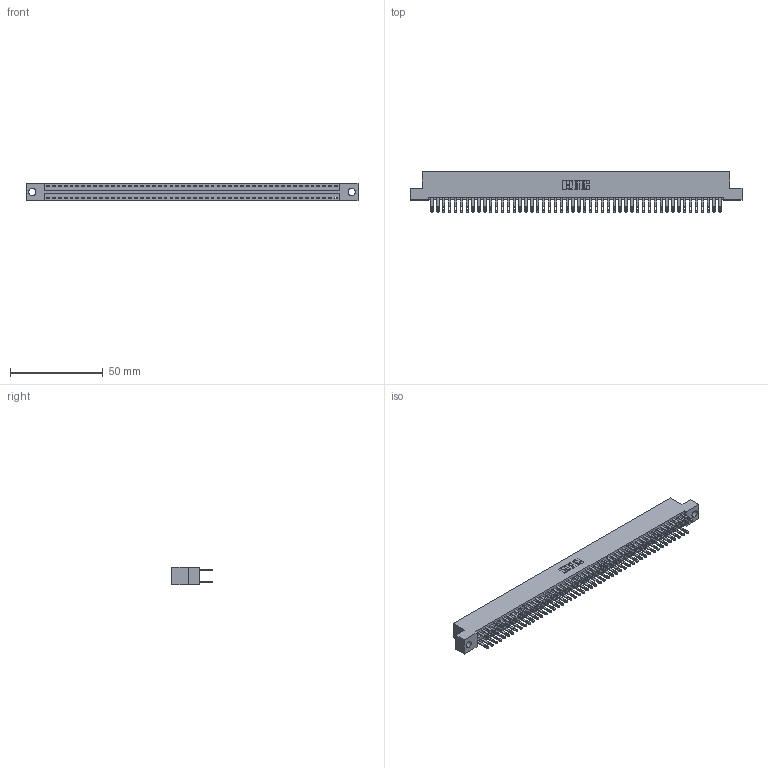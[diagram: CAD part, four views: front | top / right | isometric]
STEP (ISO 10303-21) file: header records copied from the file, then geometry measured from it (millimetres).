
FILE_DESCRIPTION (( 'STEP AP203' ), '1' );
FILE_NAME ('896-100-500-204.STEP', '2021-07-28T03:43:15', ( '' ), ( '' ), 'SwSTEP 2.0', 'SolidWorks 2020', '' );
FILE_SCHEMA (( 'CONFIG_CONTROL_DESIGN' ));
Length unit declared in the file: inch
Products named in the file (3): 345-292-001_345-293-100; 846 Part_Flush Mounting Lugs - 0.156 Dia-TH; 896-100-500-204
Assembly tree (100 placements, depth 2):
  896-100-500-204
    846 Part_Flush Mounting Lugs - 0.156 Dia-TH
    345-292-001_345-293-100  x99
Bounding box: 179.32 x 21.84 x 9.4 mm (x, y, z)
Volume: 17754.1 mm3; surface area: 25327.6 mm2
Topology: 100 solids, 100 shells, 4880 faces, 14903 edges, 9934 vertices
Faces by surface type: plane 2952, cylinder 1928
Entity records: 31455 total; most frequent: CARTESIAN_POINT 5175, ORIENTED_EDGE 5110, DIRECTION 4613, EDGE_CURVE 2555, LINE 2219, VECTOR 2219, VERTEX_POINT 1702, AXIS2_PLACEMENT_3D 1197
